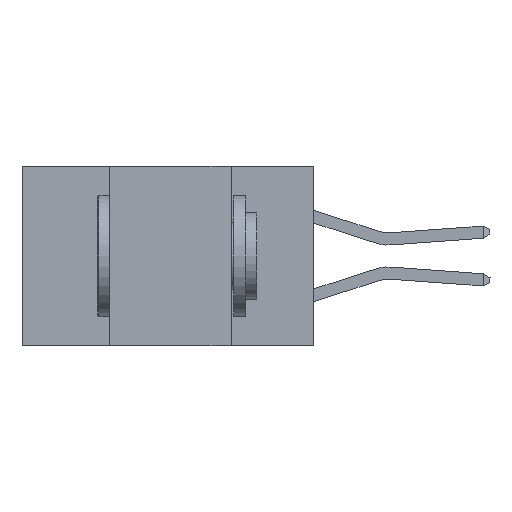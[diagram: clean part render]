
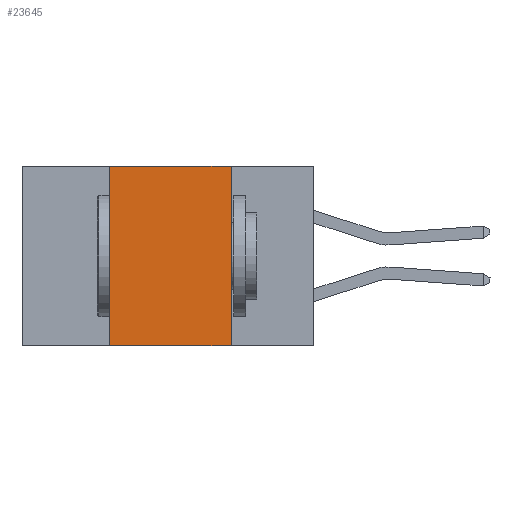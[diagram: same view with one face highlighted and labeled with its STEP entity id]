
A CAD part, left-side view. The second image highlights one B-rep face of the part: STEP entity #23645.
In plain terms, the highlighted planar face has unit normal (-1, 0, 0).
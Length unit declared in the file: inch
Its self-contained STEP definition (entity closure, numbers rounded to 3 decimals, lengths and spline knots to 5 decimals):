
#639 = VERTEX_POINT ( 'NONE', #33416 ) ;
#999 = FACE_OUTER_BOUND ( 'NONE', #31614, .T. ) ;
#2762 = PLANE ( 'NONE',  #14674 ) ;
#3970 = CARTESIAN_POINT ( 'NONE',  ( 0., 0.42, -0.37 ) ) ;
#4079 = ORIENTED_EDGE ( 'NONE', *, *, #40533, .F. ) ;
#4171 = CARTESIAN_POINT ( 'NONE',  ( 0., 0.42, 0. ) ) ;
#4439 = DIRECTION ( 'NONE',  ( 0., -1., 0. ) ) ;
#4519 = VECTOR ( 'NONE', #25968, 39.37008 ) ;
#5542 = EDGE_CURVE ( 'NONE', #41225, #639, #22684, .T. ) ;
#6689 = CARTESIAN_POINT ( 'NONE',  ( 0., 0.17, 0. ) ) ;
#7400 = VERTEX_POINT ( 'NONE', #3970 ) ;
#7609 = CARTESIAN_POINT ( 'NONE',  ( 0., 0.6, -0.37 ) ) ;
#10469 = VECTOR ( 'NONE', #27135, 39.37008 ) ;
#13198 = DIRECTION ( 'NONE',  ( 0., 0., -1. ) ) ;
#14406 = ORIENTED_EDGE ( 'NONE', *, *, #15229, .T. ) ;
#14674 = AXIS2_PLACEMENT_3D ( 'NONE', #16330, #36476, #13198 ) ;
#14708 = CARTESIAN_POINT ( 'NONE',  ( 0., 0.17, -0.37 ) ) ;
#15229 = EDGE_CURVE ( 'NONE', #7400, #38769, #28713, .T. ) ;
#16330 = CARTESIAN_POINT ( 'NONE',  ( 0., 0.6, 0. ) ) ;
#22657 = VECTOR ( 'NONE', #24923, 39.37008 ) ;
#22684 = LINE ( 'NONE', #39382, #4519 ) ;
#23645 = ADVANCED_FACE ( 'NONE', ( #999 ), #2762, .F. ) ;
#24923 = DIRECTION ( 'NONE',  ( 0., 0., 1. ) ) ;
#25968 = DIRECTION ( 'NONE',  ( 0., -1., 0. ) ) ;
#26493 = LINE ( 'NONE', #6689, #10469 ) ;
#27135 = DIRECTION ( 'NONE',  ( 0., 0., -1. ) ) ;
#27716 = ORIENTED_EDGE ( 'NONE', *, *, #5542, .F. ) ;
#27772 = CARTESIAN_POINT ( 'NONE',  ( 0., 0.42, 0. ) ) ;
#28713 = LINE ( 'NONE', #7609, #41004 ) ;
#31614 = EDGE_LOOP ( 'NONE', ( #4079, #27716, #39417, #14406 ) ) ;
#31719 = LINE ( 'NONE', #4171, #22657 ) ;
#33416 = CARTESIAN_POINT ( 'NONE',  ( 0., 0.17, 0. ) ) ;
#36476 = DIRECTION ( 'NONE',  ( 1., 0., 0. ) ) ;
#38769 = VERTEX_POINT ( 'NONE', #14708 ) ;
#39382 = CARTESIAN_POINT ( 'NONE',  ( 0., 0.6, 0. ) ) ;
#39417 = ORIENTED_EDGE ( 'NONE', *, *, #41326, .F. ) ;
#40533 = EDGE_CURVE ( 'NONE', #639, #38769, #26493, .T. ) ;
#41004 = VECTOR ( 'NONE', #4439, 39.37008 ) ;
#41225 = VERTEX_POINT ( 'NONE', #27772 ) ;
#41326 = EDGE_CURVE ( 'NONE', #7400, #41225, #31719, .T. ) ;
